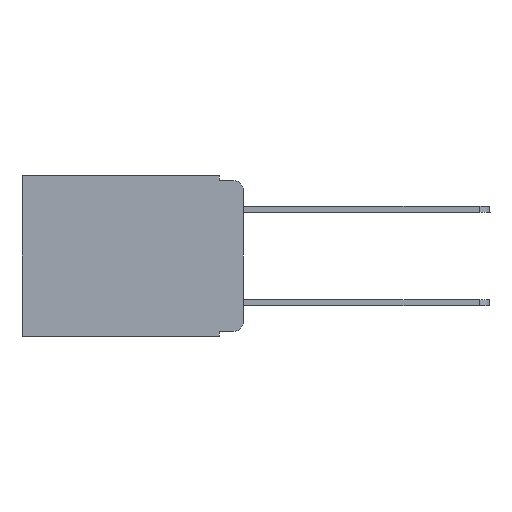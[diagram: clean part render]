
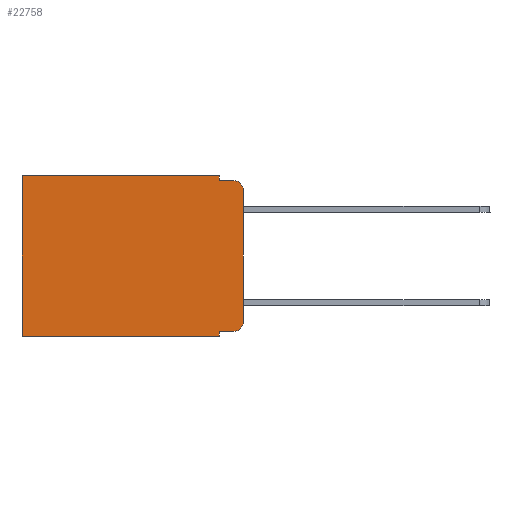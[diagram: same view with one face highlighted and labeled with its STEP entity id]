
A CAD part, left-side view. The second image highlights one B-rep face of the part: STEP entity #22758.
In plain terms, the highlighted planar face has unit normal (-1, 0, 0).
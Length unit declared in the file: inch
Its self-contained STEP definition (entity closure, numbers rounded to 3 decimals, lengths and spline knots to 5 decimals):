
#853 = CARTESIAN_POINT ( 'NONE',  ( 0.298, 0.473, 0. ) ) ;
#949 = CARTESIAN_POINT ( 'NONE',  ( 0.298, 0.051, 0. ) ) ;
#1451 = VERTEX_POINT ( 'NONE', #23940 ) ;
#2264 = VECTOR ( 'NONE', #6874, 39.37008 ) ;
#2482 = LINE ( 'NONE', #20338, #2264 ) ;
#2718 = CARTESIAN_POINT ( 'NONE',  ( 0.298, 0.473, 0. ) ) ;
#2770 = DIRECTION ( 'NONE',  ( 0., 0., -1. ) ) ;
#3187 = CARTESIAN_POINT ( 'NONE',  ( 0.298, 0.051, 0. ) ) ;
#3446 = CARTESIAN_POINT ( 'NONE',  ( 0.298, 0.051, -0.333 ) ) ;
#3676 = EDGE_CURVE ( 'NONE', #23933, #16848, #22185, .T. ) ;
#3751 = CARTESIAN_POINT ( 'NONE',  ( 0.298, 0.051, 0. ) ) ;
#4246 = CARTESIAN_POINT ( 'NONE',  ( 0.298, 0., -0.03 ) ) ;
#4291 = CARTESIAN_POINT ( 'NONE',  ( 0.298, 0.02, -0.333 ) ) ;
#4542 = EDGE_CURVE ( 'NONE', #12839, #1451, #7068, .T. ) ;
#4617 = LINE ( 'NONE', #949, #17222 ) ;
#4704 = VERTEX_POINT ( 'NONE', #3446 ) ;
#4775 = ORIENTED_EDGE ( 'NONE', *, *, #4542, .T. ) ;
#4926 = VECTOR ( 'NONE', #6678, 39.37008 ) ;
#5074 = LINE ( 'NONE', #13210, #10473 ) ;
#5526 = EDGE_CURVE ( 'NONE', #4704, #11524, #5074, .T. ) ;
#5893 = CARTESIAN_POINT ( 'NONE',  ( 0.298, 0.051, -0.01 ) ) ;
#5972 = EDGE_LOOP ( 'NONE', ( #11337, #10889, #6410, #7007, #20293, #4775, #24830, #19115, #18372, #15035 ) ) ;
#6410 = ORIENTED_EDGE ( 'NONE', *, *, #15395, .F. ) ;
#6525 = EDGE_CURVE ( 'NONE', #23933, #19464, #19749, .T. ) ;
#6678 = DIRECTION ( 'NONE',  ( 0., 0., -1. ) ) ;
#6874 = DIRECTION ( 'NONE',  ( 0., 1., 0. ) ) ;
#6993 = VECTOR ( 'NONE', #2770, 39.37008 ) ;
#7007 = ORIENTED_EDGE ( 'NONE', *, *, #10685, .F. ) ;
#7068 = LINE ( 'NONE', #853, #4926 ) ;
#7675 = VERTEX_POINT ( 'NONE', #20143 ) ;
#7918 = FACE_OUTER_BOUND ( 'NONE', #5972, .T. ) ;
#8505 = CARTESIAN_POINT ( 'NONE',  ( 0.298, 0., 0. ) ) ;
#8694 = VERTEX_POINT ( 'NONE', #3751 ) ;
#9350 = DIRECTION ( 'NONE',  ( 0., 0., -1. ) ) ;
#9725 = PLANE ( 'NONE',  #22115 ) ;
#10318 = LINE ( 'NONE', #8505, #11184 ) ;
#10473 = VECTOR ( 'NONE', #11002, 39.37008 ) ;
#10685 = EDGE_CURVE ( 'NONE', #8694, #13601, #4617, .T. ) ;
#10889 = ORIENTED_EDGE ( 'NONE', *, *, #6525, .T. ) ;
#11002 = DIRECTION ( 'NONE',  ( 0., -1., 0. ) ) ;
#11184 = VECTOR ( 'NONE', #12391, 39.37008 ) ;
#11337 = ORIENTED_EDGE ( 'NONE', *, *, #3676, .F. ) ;
#11524 = VERTEX_POINT ( 'NONE', #4291 ) ;
#11536 = VECTOR ( 'NONE', #21041, 39.37008 ) ;
#11739 = CIRCLE ( 'NONE', #23712, 0.02 ) ;
#12178 = DIRECTION ( 'NONE',  ( 1., 0., 0. ) ) ;
#12391 = DIRECTION ( 'NONE',  ( 0., 1., 0. ) ) ;
#12839 = VERTEX_POINT ( 'NONE', #2718 ) ;
#13210 = CARTESIAN_POINT ( 'NONE',  ( 0.298, 0.051, -0.333 ) ) ;
#13601 = VERTEX_POINT ( 'NONE', #5893 ) ;
#14058 = LINE ( 'NONE', #3187, #11536 ) ;
#14687 = DIRECTION ( 'NONE',  ( 0., 0., -1. ) ) ;
#14938 = CARTESIAN_POINT ( 'NONE',  ( 0.298, 0., -0.313 ) ) ;
#15035 = ORIENTED_EDGE ( 'NONE', *, *, #22604, .T. ) ;
#15075 = EDGE_CURVE ( 'NONE', #4704, #7675, #14058, .T. ) ;
#15395 = EDGE_CURVE ( 'NONE', #13601, #19464, #22531, .T. ) ;
#15545 = CARTESIAN_POINT ( 'NONE',  ( 0.298, 0.02, -0.313 ) ) ;
#15676 = CARTESIAN_POINT ( 'NONE',  ( 0.298, 0., 0. ) ) ;
#16098 = CARTESIAN_POINT ( 'NONE',  ( 0.298, 0.051, -0.01 ) ) ;
#16848 = VERTEX_POINT ( 'NONE', #14938 ) ;
#16871 = AXIS2_PLACEMENT_3D ( 'NONE', #21264, #25274, #23319 ) ;
#17222 = VECTOR ( 'NONE', #14687, 39.37008 ) ;
#17591 = EDGE_CURVE ( 'NONE', #8694, #12839, #10318, .T. ) ;
#17626 = DIRECTION ( 'NONE',  ( 0., 0., -1. ) ) ;
#17911 = DIRECTION ( 'NONE',  ( 0., -1., 0. ) ) ;
#18372 = ORIENTED_EDGE ( 'NONE', *, *, #5526, .T. ) ;
#19115 = ORIENTED_EDGE ( 'NONE', *, *, #15075, .F. ) ;
#19464 = VERTEX_POINT ( 'NONE', #25294 ) ;
#19749 = CIRCLE ( 'NONE', #16871, 0.02 ) ;
#20143 = CARTESIAN_POINT ( 'NONE',  ( 0.298, 0.051, -0.343 ) ) ;
#20293 = ORIENTED_EDGE ( 'NONE', *, *, #17591, .T. ) ;
#20338 = CARTESIAN_POINT ( 'NONE',  ( 0.298, 0., -0.343 ) ) ;
#21041 = DIRECTION ( 'NONE',  ( 0., 0., -1. ) ) ;
#21264 = CARTESIAN_POINT ( 'NONE',  ( 0.298, 0.02, -0.03 ) ) ;
#21890 = VECTOR ( 'NONE', #17911, 39.37008 ) ;
#22115 = AXIS2_PLACEMENT_3D ( 'NONE', #15676, #12178, #17626 ) ;
#22185 = LINE ( 'NONE', #22435, #6993 ) ;
#22435 = CARTESIAN_POINT ( 'NONE',  ( 0.298, 0., 0. ) ) ;
#22531 = LINE ( 'NONE', #16098, #21890 ) ;
#22604 = EDGE_CURVE ( 'NONE', #11524, #16848, #11739, .T. ) ;
#22758 = ADVANCED_FACE ( 'NONE', ( #7918 ), #9725, .F. ) ;
#22884 = EDGE_CURVE ( 'NONE', #7675, #1451, #2482, .T. ) ;
#23311 = DIRECTION ( 'NONE',  ( -1., 0., 0. ) ) ;
#23319 = DIRECTION ( 'NONE',  ( 0., 0., -1. ) ) ;
#23712 = AXIS2_PLACEMENT_3D ( 'NONE', #15545, #23311, #9350 ) ;
#23933 = VERTEX_POINT ( 'NONE', #4246 ) ;
#23940 = CARTESIAN_POINT ( 'NONE',  ( 0.298, 0.473, -0.343 ) ) ;
#24830 = ORIENTED_EDGE ( 'NONE', *, *, #22884, .F. ) ;
#25274 = DIRECTION ( 'NONE',  ( -1., 0., 0. ) ) ;
#25294 = CARTESIAN_POINT ( 'NONE',  ( 0.298, 0.02, -0.01 ) ) ;
